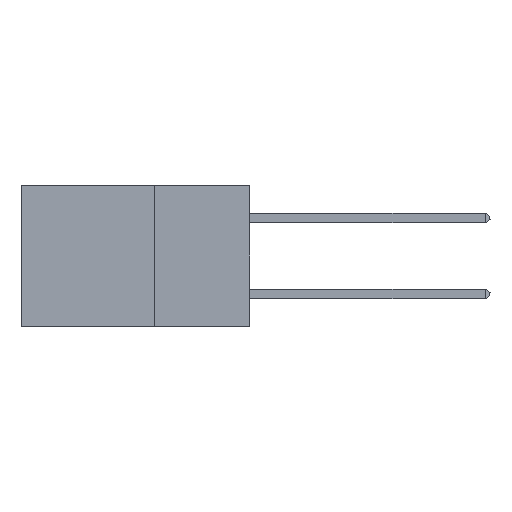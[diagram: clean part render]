
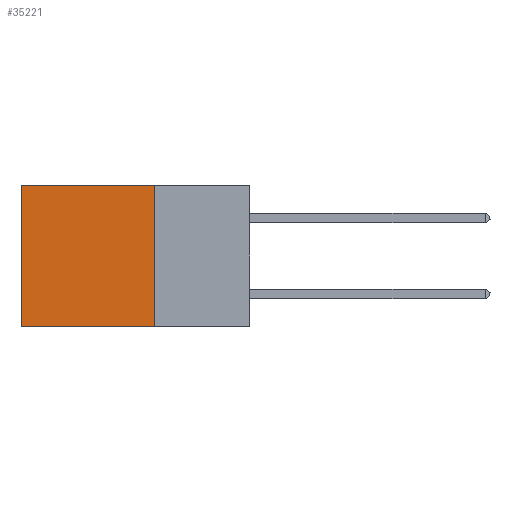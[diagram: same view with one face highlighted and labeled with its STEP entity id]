
A CAD part, left-side view. The second image highlights one B-rep face of the part: STEP entity #35221.
In plain terms, the highlighted planar face has unit normal (-1, 0, 0).
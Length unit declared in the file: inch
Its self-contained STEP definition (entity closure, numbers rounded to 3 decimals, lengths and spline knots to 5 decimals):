
#380 = LINE ( 'NONE', #31481, #7314 ) ;
#2809 = VERTEX_POINT ( 'NONE', #21102 ) ;
#3901 = LINE ( 'NONE', #20568, #10761 ) ;
#5483 = VECTOR ( 'NONE', #33632, 39.37008 ) ;
#6024 = DIRECTION ( 'NONE',  ( 0., 0., -1. ) ) ;
#6062 = LINE ( 'NONE', #24839, #35774 ) ;
#6172 = DIRECTION ( 'NONE',  ( 1., 0., 0. ) ) ;
#7037 = ORIENTED_EDGE ( 'NONE', *, *, #32753, .F. ) ;
#7314 = VECTOR ( 'NONE', #8474, 39.37008 ) ;
#7741 = CARTESIAN_POINT ( 'NONE',  ( 0.2875, 0.25, 0. ) ) ;
#8474 = DIRECTION ( 'NONE',  ( 0., 1., 0. ) ) ;
#10074 = VERTEX_POINT ( 'NONE', #29155 ) ;
#10761 = VECTOR ( 'NONE', #6024, 39.37008 ) ;
#13333 = ORIENTED_EDGE ( 'NONE', *, *, #19925, .T. ) ;
#13362 = CARTESIAN_POINT ( 'NONE',  ( 0.2875, 0.6, -0.37 ) ) ;
#14776 = EDGE_CURVE ( 'NONE', #10074, #29983, #380, .T. ) ;
#15574 = CARTESIAN_POINT ( 'NONE',  ( 0.2875, 0.25, 0. ) ) ;
#15717 = VERTEX_POINT ( 'NONE', #15574 ) ;
#17810 = FACE_OUTER_BOUND ( 'NONE', #31740, .T. ) ;
#19925 = EDGE_CURVE ( 'NONE', #2809, #29983, #3901, .T. ) ;
#20568 = CARTESIAN_POINT ( 'NONE',  ( 0.2875, 0.6, 0. ) ) ;
#20594 = CARTESIAN_POINT ( 'NONE',  ( 0.2875, 0.25, 0. ) ) ;
#21102 = CARTESIAN_POINT ( 'NONE',  ( 0.2875, 0.6, 0. ) ) ;
#23594 = PLANE ( 'NONE',  #34110 ) ;
#24839 = CARTESIAN_POINT ( 'NONE',  ( 0.2875, 0.25, 0. ) ) ;
#26461 = DIRECTION ( 'NONE',  ( 0., 0., -1. ) ) ;
#27704 = DIRECTION ( 'NONE',  ( 0., 0., -1. ) ) ;
#28259 = ORIENTED_EDGE ( 'NONE', *, *, #34934, .T. ) ;
#28569 = LINE ( 'NONE', #7741, #5483 ) ;
#28636 = ORIENTED_EDGE ( 'NONE', *, *, #14776, .F. ) ;
#29155 = CARTESIAN_POINT ( 'NONE',  ( 0.2875, 0.25, -0.37 ) ) ;
#29983 = VERTEX_POINT ( 'NONE', #13362 ) ;
#31481 = CARTESIAN_POINT ( 'NONE',  ( 0.2875, 0.25, -0.37 ) ) ;
#31740 = EDGE_LOOP ( 'NONE', ( #13333, #28636, #7037, #28259 ) ) ;
#32753 = EDGE_CURVE ( 'NONE', #15717, #10074, #6062, .T. ) ;
#33632 = DIRECTION ( 'NONE',  ( 0., 1., 0. ) ) ;
#34110 = AXIS2_PLACEMENT_3D ( 'NONE', #20594, #6172, #26461 ) ;
#34934 = EDGE_CURVE ( 'NONE', #15717, #2809, #28569, .T. ) ;
#35221 = ADVANCED_FACE ( 'NONE', ( #17810 ), #23594, .F. ) ;
#35774 = VECTOR ( 'NONE', #27704, 39.37008 ) ;
